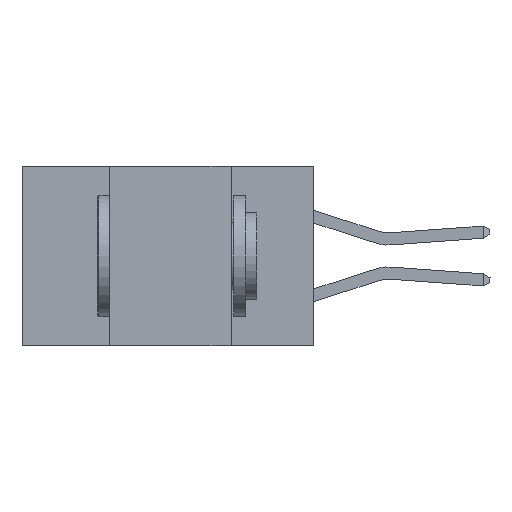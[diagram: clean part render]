
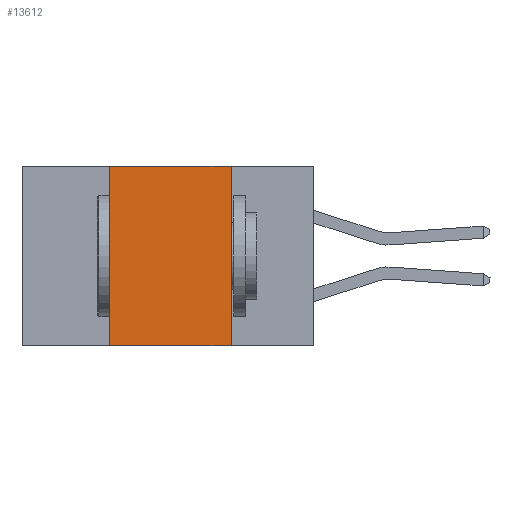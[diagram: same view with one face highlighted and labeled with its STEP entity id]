
A CAD part, left-side view. The second image highlights one B-rep face of the part: STEP entity #13612.
In plain terms, the highlighted planar face has unit normal (-1, 0, 0).
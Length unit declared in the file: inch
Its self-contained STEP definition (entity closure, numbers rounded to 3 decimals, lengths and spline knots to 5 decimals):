
#150 = CARTESIAN_POINT ( 'NONE',  ( 0., 0.42, 0. ) ) ;
#540 = EDGE_CURVE ( 'NONE', #6376, #8075, #3836, .T. ) ;
#1415 = CARTESIAN_POINT ( 'NONE',  ( 0., 0.42, -0.37 ) ) ;
#2552 = ORIENTED_EDGE ( 'NONE', *, *, #15804, .F. ) ;
#2618 = ORIENTED_EDGE ( 'NONE', *, *, #6322, .F. ) ;
#2925 = CARTESIAN_POINT ( 'NONE',  ( 0., 0.6, -0.37 ) ) ;
#3836 = LINE ( 'NONE', #10896, #20377 ) ;
#4272 = PLANE ( 'NONE',  #16733 ) ;
#4354 = ORIENTED_EDGE ( 'NONE', *, *, #6060, .T. ) ;
#4674 = EDGE_LOOP ( 'NONE', ( #15621, #2552, #2618, #4354 ) ) ;
#4934 = DIRECTION ( 'NONE',  ( 0., -1., 0. ) ) ;
#6060 = EDGE_CURVE ( 'NONE', #7207, #8075, #20759, .T. ) ;
#6322 = EDGE_CURVE ( 'NONE', #7207, #12139, #19495, .T. ) ;
#6376 = VERTEX_POINT ( 'NONE', #16536 ) ;
#7207 = VERTEX_POINT ( 'NONE', #1415 ) ;
#8075 = VERTEX_POINT ( 'NONE', #19790 ) ;
#9137 = DIRECTION ( 'NONE',  ( 1., 0., 0. ) ) ;
#10481 = DIRECTION ( 'NONE',  ( 0., 0., -1. ) ) ;
#10896 = CARTESIAN_POINT ( 'NONE',  ( 0., 0.17, 0. ) ) ;
#11021 = VECTOR ( 'NONE', #17975, 39.37008 ) ;
#11376 = CARTESIAN_POINT ( 'NONE',  ( 0., 0.6, 0. ) ) ;
#12139 = VERTEX_POINT ( 'NONE', #150 ) ;
#13612 = ADVANCED_FACE ( 'NONE', ( #18537 ), #4272, .F. ) ;
#14982 = LINE ( 'NONE', #11376, #18714 ) ;
#15621 = ORIENTED_EDGE ( 'NONE', *, *, #540, .F. ) ;
#15769 = DIRECTION ( 'NONE',  ( 0., -1., 0. ) ) ;
#15804 = EDGE_CURVE ( 'NONE', #12139, #6376, #14982, .T. ) ;
#16033 = VECTOR ( 'NONE', #15769, 39.37008 ) ;
#16536 = CARTESIAN_POINT ( 'NONE',  ( 0., 0.17, 0. ) ) ;
#16733 = AXIS2_PLACEMENT_3D ( 'NONE', #18717, #9137, #20322 ) ;
#17975 = DIRECTION ( 'NONE',  ( 0., 0., 1. ) ) ;
#18537 = FACE_OUTER_BOUND ( 'NONE', #4674, .T. ) ;
#18714 = VECTOR ( 'NONE', #4934, 39.37008 ) ;
#18717 = CARTESIAN_POINT ( 'NONE',  ( 0., 0.6, 0. ) ) ;
#19495 = LINE ( 'NONE', #19570, #11021 ) ;
#19570 = CARTESIAN_POINT ( 'NONE',  ( 0., 0.42, 0. ) ) ;
#19790 = CARTESIAN_POINT ( 'NONE',  ( 0., 0.17, -0.37 ) ) ;
#20322 = DIRECTION ( 'NONE',  ( 0., 0., -1. ) ) ;
#20377 = VECTOR ( 'NONE', #10481, 39.37008 ) ;
#20759 = LINE ( 'NONE', #2925, #16033 ) ;
